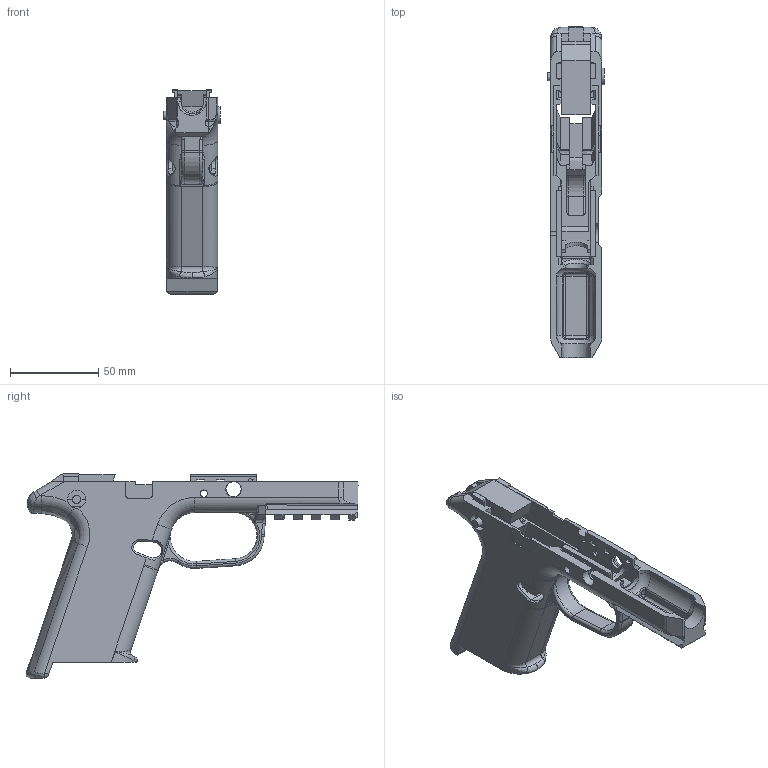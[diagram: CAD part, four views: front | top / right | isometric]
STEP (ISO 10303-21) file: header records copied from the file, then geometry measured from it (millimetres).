
FILE_DESCRIPTION(/* description */ (''),/* implementation_level */ '2;1');
FILE_NAME(/* name */ 'FNX.step',/* time_stamp */ '2022-03-03T23:43:30-05:00',/* author */ (''),/* organization */ (''),/* preprocessor_version */ 'ST-DEVELOPER v18.1',/* originating_system */ 'Autodesk Translation Framework v10.13.0.1454',/* authorisation */ '');
FILE_SCHEMA (('AUTOMOTIVE_DESIGN { 1 0 10303 214 3 1 1 }'));
Length unit declared in the file: millimetre
Products named in the file (10): FNX; FNX Frame; Left-hand Rail Plate; Right-hand Rail Plate; Right-hand Front Rail Plate; Left-hand Front Rail Plate; Center Front Rail Plate; Hammer Housing; Safety Lever; Frame
Assembly tree (9 placements, depth 3):
  FNX
    FNX Frame
      Left-hand Rail Plate
      Right-hand Rail Plate
      Right-hand Front Rail Plate
      Left-hand Front Rail Plate
      Center Front Rail Plate
      Hammer Housing
      Safety Lever
      Frame
Bounding box: 31.8 x 188.27 x 115.75 mm (x, y, z)
Volume: 110876.6 mm3; surface area: 58354.6 mm2
Topology: 8 solids, 8 shells, 614 faces, 1720 edges, 1106 vertices
Faces by surface type: plane 389, bspline 103, cylinder 93, torus 22, sphere 4, cone 3
Full cylindrical faces by diameter (mm): 4.05 x4, 4.65 x1, 4.7 x2, 4.76 x2, 8.52 x2, 9.5 x1, 10.2 x2
Entity records: 23437 total; most frequent: CARTESIAN_POINT 7854, ORIENTED_EDGE 3430, DIRECTION 2825, EDGE_CURVE 1715, LINE 1179, VECTOR 1179, VERTEX_POINT 1106, AXIS2_PLACEMENT_3D 823
